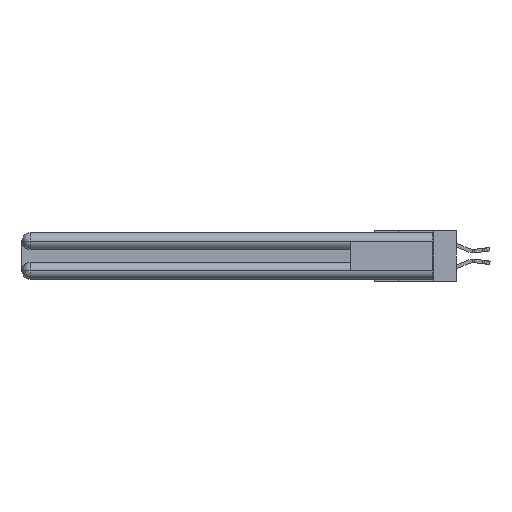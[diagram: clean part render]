
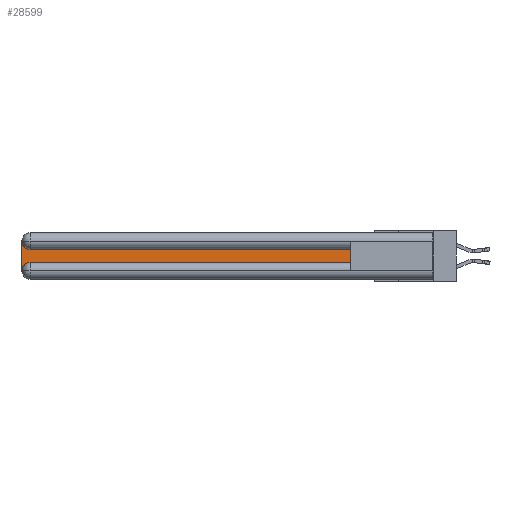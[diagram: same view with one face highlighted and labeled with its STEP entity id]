
A CAD part, left-side view. The second image highlights one B-rep face of the part: STEP entity #28599.
In plain terms, the highlighted planar face has unit normal (-1, 0, 0).
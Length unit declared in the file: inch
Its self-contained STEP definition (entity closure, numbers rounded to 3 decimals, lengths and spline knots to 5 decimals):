
#189 = CARTESIAN_POINT ( 'NONE',  ( 0.075, 0.6, -0.2175 ) ) ;
#853 = CIRCLE ( 'NONE', #8644, 0.06 ) ;
#1078 = VERTEX_POINT ( 'NONE', #13710 ) ;
#1257 = FACE_OUTER_BOUND ( 'NONE', #26768, .T. ) ;
#1276 = VERTEX_POINT ( 'NONE', #14780 ) ;
#1511 = ORIENTED_EDGE ( 'NONE', *, *, #13686, .T. ) ;
#1907 = CARTESIAN_POINT ( 'NONE',  ( 0.075, 3., -0.2175 ) ) ;
#2881 = LINE ( 'NONE', #189, #27193 ) ;
#2895 = VERTEX_POINT ( 'NONE', #5483 ) ;
#3083 = PLANE ( 'NONE',  #8830 ) ;
#3517 = ORIENTED_EDGE ( 'NONE', *, *, #5015, .T. ) ;
#4213 = DIRECTION ( 'NONE',  ( 0., 0., -1. ) ) ;
#5015 = EDGE_CURVE ( 'NONE', #13093, #2895, #2881, .T. ) ;
#5483 = CARTESIAN_POINT ( 'NONE',  ( 0.075, 0.6, -0.2175 ) ) ;
#5843 = CIRCLE ( 'NONE', #23962, 0.06 ) ;
#5989 = VERTEX_POINT ( 'NONE', #24306 ) ;
#6265 = DIRECTION ( 'NONE',  ( 0., 1., 0. ) ) ;
#7379 = VERTEX_POINT ( 'NONE', #19806 ) ;
#7679 = DIRECTION ( 'NONE',  ( 1., 0., 0. ) ) ;
#7867 = CARTESIAN_POINT ( 'NONE',  ( 0.075, 0.6, -0.1225 ) ) ;
#8644 = AXIS2_PLACEMENT_3D ( 'NONE', #19981, #26919, #4213 ) ;
#8830 = AXIS2_PLACEMENT_3D ( 'NONE', #27969, #16880, #18850 ) ;
#8952 = ORIENTED_EDGE ( 'NONE', *, *, #21799, .T. ) ;
#9148 = DIRECTION ( 'NONE',  ( 0., 0., 1. ) ) ;
#10042 = LINE ( 'NONE', #1907, #15681 ) ;
#10214 = DIRECTION ( 'NONE',  ( 0., 0., -1. ) ) ;
#10917 = ORIENTED_EDGE ( 'NONE', *, *, #13191, .T. ) ;
#11100 = DIRECTION ( 'NONE',  ( 0., 0., -1. ) ) ;
#11227 = EDGE_CURVE ( 'NONE', #1078, #5989, #10042, .T. ) ;
#13093 = VERTEX_POINT ( 'NONE', #28801 ) ;
#13191 = EDGE_CURVE ( 'NONE', #5989, #13093, #853, .T. ) ;
#13686 = EDGE_CURVE ( 'NONE', #1276, #7379, #29080, .T. ) ;
#13710 = CARTESIAN_POINT ( 'NONE',  ( 0.075, 3., -0.0625 ) ) ;
#14266 = CARTESIAN_POINT ( 'NONE',  ( 0.075, 2.94, -0.0625 ) ) ;
#14780 = CARTESIAN_POINT ( 'NONE',  ( 0.075, 0.6, -0.1225 ) ) ;
#15681 = VECTOR ( 'NONE', #11100, 39.37008 ) ;
#16067 = DIRECTION ( 'NONE',  ( 0., -1., 0. ) ) ;
#16880 = DIRECTION ( 'NONE',  ( 1., 0., 0. ) ) ;
#18096 = CARTESIAN_POINT ( 'NONE',  ( 0.075, 0.6, -0.2175 ) ) ;
#18850 = DIRECTION ( 'NONE',  ( 0., 0., -1. ) ) ;
#18854 = LINE ( 'NONE', #18096, #27619 ) ;
#19045 = ORIENTED_EDGE ( 'NONE', *, *, #11227, .T. ) ;
#19806 = CARTESIAN_POINT ( 'NONE',  ( 0.075, 2.94, -0.1225 ) ) ;
#19981 = CARTESIAN_POINT ( 'NONE',  ( 0.075, 2.94, -0.2775 ) ) ;
#21799 = EDGE_CURVE ( 'NONE', #2895, #1276, #18854, .T. ) ;
#23962 = AXIS2_PLACEMENT_3D ( 'NONE', #14266, #7679, #10214 ) ;
#23995 = EDGE_CURVE ( 'NONE', #7379, #1078, #5843, .T. ) ;
#24306 = CARTESIAN_POINT ( 'NONE',  ( 0.075, 3., -0.2775 ) ) ;
#26768 = EDGE_LOOP ( 'NONE', ( #1511, #27945, #19045, #10917, #3517, #8952 ) ) ;
#26919 = DIRECTION ( 'NONE',  ( 1., 0., 0. ) ) ;
#27193 = VECTOR ( 'NONE', #16067, 39.37008 ) ;
#27619 = VECTOR ( 'NONE', #9148, 39.37008 ) ;
#27945 = ORIENTED_EDGE ( 'NONE', *, *, #23995, .T. ) ;
#27969 = CARTESIAN_POINT ( 'NONE',  ( 0.075, 3., -0.1225 ) ) ;
#28382 = VECTOR ( 'NONE', #6265, 39.37008 ) ;
#28599 = ADVANCED_FACE ( 'NONE', ( #1257 ), #3083, .F. ) ;
#28801 = CARTESIAN_POINT ( 'NONE',  ( 0.075, 2.94, -0.2175 ) ) ;
#29080 = LINE ( 'NONE', #7867, #28382 ) ;
